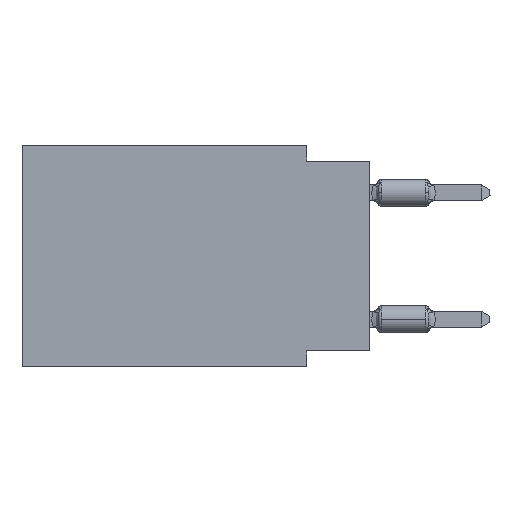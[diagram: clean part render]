
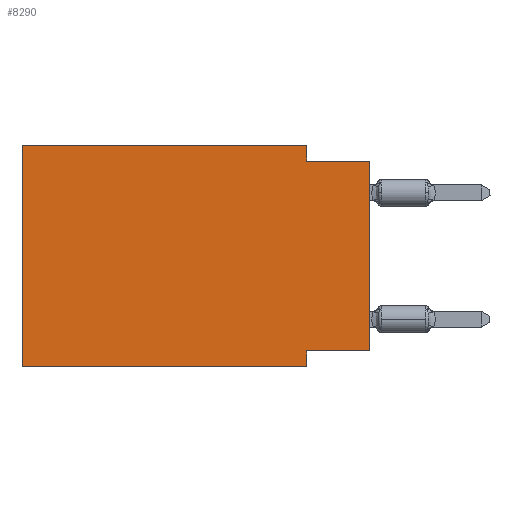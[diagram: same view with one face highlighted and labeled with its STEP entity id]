
A CAD part, left-side view. The second image highlights one B-rep face of the part: STEP entity #8290.
In plain terms, the highlighted planar face has unit normal (-1, 0, 0).
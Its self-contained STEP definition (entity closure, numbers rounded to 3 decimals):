
#285 = CARTESIAN_POINT ( 'NONE',  ( 0., 13.97, 0. ) ) ;
#428 = CARTESIAN_POINT ( 'NONE',  ( 0., 0., -8.255 ) ) ;
#1342 = EDGE_CURVE ( 'NONE', #17930, #9468, #13443, .T. ) ;
#1625 = ORIENTED_EDGE ( 'NONE', *, *, #1342, .F. ) ;
#2951 = EDGE_CURVE ( 'NONE', #4891, #17849, #7572, .T. ) ;
#3543 = LINE ( 'NONE', #20872, #11577 ) ;
#4822 = VECTOR ( 'NONE', #30970, 1000. ) ;
#4891 = VERTEX_POINT ( 'NONE', #13876 ) ;
#4941 = VECTOR ( 'NONE', #8570, 1000. ) ;
#7431 = DIRECTION ( 'NONE',  ( 0., -1., 0. ) ) ;
#7572 = LINE ( 'NONE', #285, #16893 ) ;
#7834 = CARTESIAN_POINT ( 'NONE',  ( 0., 13.97, 0. ) ) ;
#8290 = ADVANCED_FACE ( 'NONE', ( #9312 ), #26789, .F. ) ;
#8570 = DIRECTION ( 'NONE',  ( 0., -1., 0. ) ) ;
#8938 = CARTESIAN_POINT ( 'NONE',  ( 0., 13.97, 0. ) ) ;
#9190 = CARTESIAN_POINT ( 'NONE',  ( 0., 0., -0.635 ) ) ;
#9312 = FACE_OUTER_BOUND ( 'NONE', #14055, .T. ) ;
#9468 = VERTEX_POINT ( 'NONE', #9190 ) ;
#9659 = CARTESIAN_POINT ( 'NONE',  ( 0., 0., -8.255 ) ) ;
#11046 = EDGE_CURVE ( 'NONE', #11110, #22720, #21819, .T. ) ;
#11076 = VECTOR ( 'NONE', #7431, 1000. ) ;
#11110 = VERTEX_POINT ( 'NONE', #428 ) ;
#11524 = EDGE_CURVE ( 'NONE', #17849, #14462, #14816, .T. ) ;
#11577 = VECTOR ( 'NONE', #30736, 1000. ) ;
#12111 = EDGE_CURVE ( 'NONE', #14462, #17930, #23781, .T. ) ;
#12667 = CARTESIAN_POINT ( 'NONE',  ( 0., 2.54, 0. ) ) ;
#13443 = LINE ( 'NONE', #15872, #4941 ) ;
#13686 = EDGE_CURVE ( 'NONE', #4891, #15105, #19752, .T. ) ;
#13784 = CARTESIAN_POINT ( 'NONE',  ( 0., 2.54, -8.255 ) ) ;
#13876 = CARTESIAN_POINT ( 'NONE',  ( 0., 13.97, -8.89 ) ) ;
#14055 = EDGE_LOOP ( 'NONE', ( #31697, #1625, #20523, #25917, #22842, #24908, #25710, #26654 ) ) ;
#14462 = VERTEX_POINT ( 'NONE', #12667 ) ;
#14816 = LINE ( 'NONE', #7834, #25010 ) ;
#15105 = VERTEX_POINT ( 'NONE', #19164 ) ;
#15859 = DIRECTION ( 'NONE',  ( 0., 0., -1. ) ) ;
#15872 = CARTESIAN_POINT ( 'NONE',  ( 0., 0., -0.635 ) ) ;
#16549 = AXIS2_PLACEMENT_3D ( 'NONE', #21936, #31789, #24045 ) ;
#16559 = LINE ( 'NONE', #21109, #4822 ) ;
#16893 = VECTOR ( 'NONE', #20374, 1000. ) ;
#17849 = VERTEX_POINT ( 'NONE', #8938 ) ;
#17930 = VERTEX_POINT ( 'NONE', #18976 ) ;
#18911 = DIRECTION ( 'NONE',  ( 0., 1., 0. ) ) ;
#18976 = CARTESIAN_POINT ( 'NONE',  ( 0., 2.54, -0.635 ) ) ;
#19164 = CARTESIAN_POINT ( 'NONE',  ( 0., 2.54, -8.89 ) ) ;
#19277 = VECTOR ( 'NONE', #15859, 1000. ) ;
#19752 = LINE ( 'NONE', #29611, #11076 ) ;
#20293 = VECTOR ( 'NONE', #18911, 1000. ) ;
#20374 = DIRECTION ( 'NONE',  ( 0., 0., 1. ) ) ;
#20523 = ORIENTED_EDGE ( 'NONE', *, *, #12111, .F. ) ;
#20872 = CARTESIAN_POINT ( 'NONE',  ( 0., 0., 0. ) ) ;
#21109 = CARTESIAN_POINT ( 'NONE',  ( 0., 2.54, -8.89 ) ) ;
#21819 = LINE ( 'NONE', #9659, #20293 ) ;
#21936 = CARTESIAN_POINT ( 'NONE',  ( 0., 13.97, 0. ) ) ;
#22098 = EDGE_CURVE ( 'NONE', #22720, #15105, #16559, .T. ) ;
#22720 = VERTEX_POINT ( 'NONE', #13784 ) ;
#22842 = ORIENTED_EDGE ( 'NONE', *, *, #2951, .F. ) ;
#23204 = EDGE_CURVE ( 'NONE', #11110, #9468, #3543, .T. ) ;
#23781 = LINE ( 'NONE', #28467, #19277 ) ;
#24045 = DIRECTION ( 'NONE',  ( 0., 0., -1. ) ) ;
#24908 = ORIENTED_EDGE ( 'NONE', *, *, #13686, .T. ) ;
#25010 = VECTOR ( 'NONE', #29851, 1000. ) ;
#25710 = ORIENTED_EDGE ( 'NONE', *, *, #22098, .F. ) ;
#25917 = ORIENTED_EDGE ( 'NONE', *, *, #11524, .F. ) ;
#26654 = ORIENTED_EDGE ( 'NONE', *, *, #11046, .F. ) ;
#26789 = PLANE ( 'NONE',  #16549 ) ;
#28467 = CARTESIAN_POINT ( 'NONE',  ( 0., 2.54, 0. ) ) ;
#29611 = CARTESIAN_POINT ( 'NONE',  ( 0., 13.97, -8.89 ) ) ;
#29851 = DIRECTION ( 'NONE',  ( 0., -1., 0. ) ) ;
#30736 = DIRECTION ( 'NONE',  ( 0., 0., 1. ) ) ;
#30970 = DIRECTION ( 'NONE',  ( 0., 0., -1. ) ) ;
#31697 = ORIENTED_EDGE ( 'NONE', *, *, #23204, .T. ) ;
#31789 = DIRECTION ( 'NONE',  ( 1., 0., 0. ) ) ;
